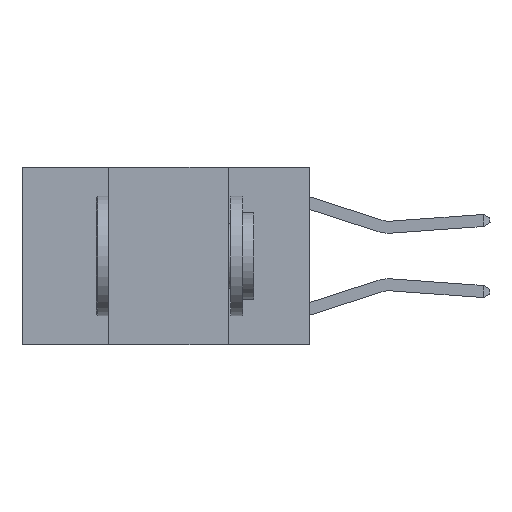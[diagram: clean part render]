
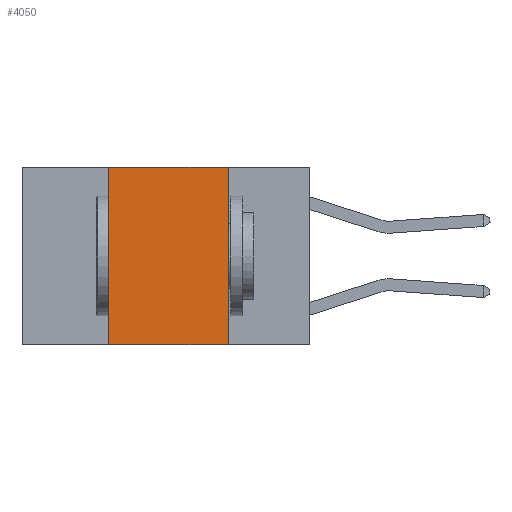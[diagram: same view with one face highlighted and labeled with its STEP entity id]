
A CAD part, left-side view. The second image highlights one B-rep face of the part: STEP entity #4050.
In plain terms, the highlighted planar face has unit normal (-1, 0, 0).
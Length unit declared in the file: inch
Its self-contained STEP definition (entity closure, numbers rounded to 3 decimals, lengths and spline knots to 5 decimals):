
#255 = EDGE_CURVE ( 'NONE', #7324, #3226, #4578, .T. ) ;
#477 = DIRECTION ( 'NONE',  ( 1., 0., 0. ) ) ;
#645 = CARTESIAN_POINT ( 'NONE',  ( 0., 0.17, -0.37 ) ) ;
#1634 = VECTOR ( 'NONE', #9570, 39.37008 ) ;
#1706 = VECTOR ( 'NONE', #10311, 39.37008 ) ;
#2014 = CARTESIAN_POINT ( 'NONE',  ( 0., 0.17, 0. ) ) ;
#2165 = DIRECTION ( 'NONE',  ( 0., -1., 0. ) ) ;
#2238 = EDGE_LOOP ( 'NONE', ( #3801, #5005, #10902, #13653 ) ) ;
#2421 = AXIS2_PLACEMENT_3D ( 'NONE', #6886, #477, #8021 ) ;
#3226 = VERTEX_POINT ( 'NONE', #7807 ) ;
#3750 = EDGE_CURVE ( 'NONE', #10983, #7289, #5969, .T. ) ;
#3801 = ORIENTED_EDGE ( 'NONE', *, *, #8914, .F. ) ;
#3866 = CARTESIAN_POINT ( 'NONE',  ( 0., 0.42, 0. ) ) ;
#4050 = ADVANCED_FACE ( 'NONE', ( #12959 ), #4735, .F. ) ;
#4098 = CARTESIAN_POINT ( 'NONE',  ( 0., 0.6, 0. ) ) ;
#4196 = DIRECTION ( 'NONE',  ( 0., 0., 1. ) ) ;
#4476 = VECTOR ( 'NONE', #4196, 39.37008 ) ;
#4578 = LINE ( 'NONE', #4098, #1706 ) ;
#4735 = PLANE ( 'NONE',  #2421 ) ;
#5005 = ORIENTED_EDGE ( 'NONE', *, *, #255, .F. ) ;
#5361 = CARTESIAN_POINT ( 'NONE',  ( 0., 0.6, -0.37 ) ) ;
#5969 = LINE ( 'NONE', #5361, #13460 ) ;
#6886 = CARTESIAN_POINT ( 'NONE',  ( 0., 0.6, 0. ) ) ;
#7289 = VERTEX_POINT ( 'NONE', #645 ) ;
#7324 = VERTEX_POINT ( 'NONE', #3866 ) ;
#7341 = LINE ( 'NONE', #10637, #4476 ) ;
#7807 = CARTESIAN_POINT ( 'NONE',  ( 0., 0.17, 0. ) ) ;
#8021 = DIRECTION ( 'NONE',  ( 0., 0., -1. ) ) ;
#8914 = EDGE_CURVE ( 'NONE', #3226, #7289, #9574, .T. ) ;
#9570 = DIRECTION ( 'NONE',  ( 0., 0., -1. ) ) ;
#9574 = LINE ( 'NONE', #2014, #1634 ) ;
#10311 = DIRECTION ( 'NONE',  ( 0., -1., 0. ) ) ;
#10637 = CARTESIAN_POINT ( 'NONE',  ( 0., 0.42, 0. ) ) ;
#10902 = ORIENTED_EDGE ( 'NONE', *, *, #11241, .F. ) ;
#10983 = VERTEX_POINT ( 'NONE', #11237 ) ;
#11237 = CARTESIAN_POINT ( 'NONE',  ( 0., 0.42, -0.37 ) ) ;
#11241 = EDGE_CURVE ( 'NONE', #10983, #7324, #7341, .T. ) ;
#12959 = FACE_OUTER_BOUND ( 'NONE', #2238, .T. ) ;
#13460 = VECTOR ( 'NONE', #2165, 39.37008 ) ;
#13653 = ORIENTED_EDGE ( 'NONE', *, *, #3750, .T. ) ;
